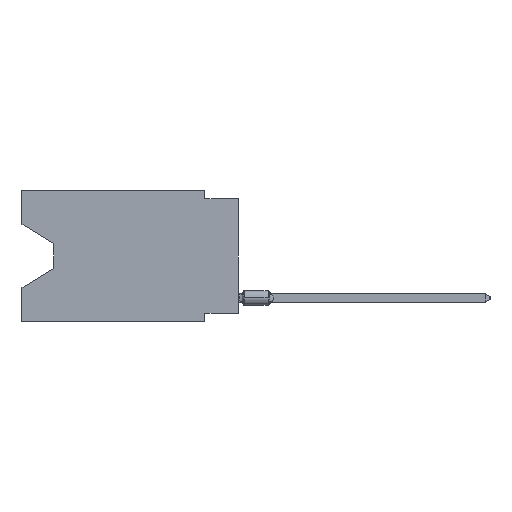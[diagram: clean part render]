
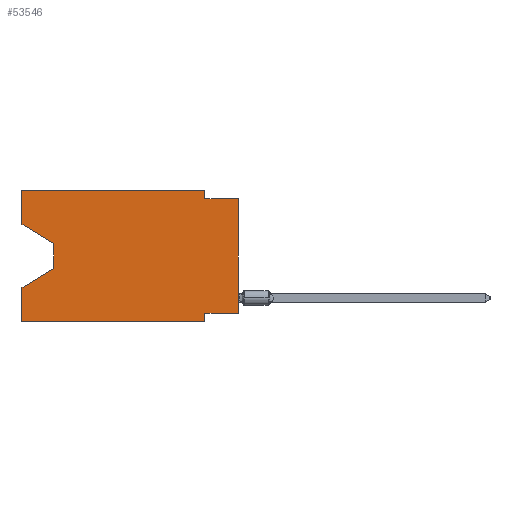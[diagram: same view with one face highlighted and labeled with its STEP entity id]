
A CAD part, left-side view. The second image highlights one B-rep face of the part: STEP entity #53546.
In plain terms, the highlighted planar face has unit normal (-1, 0, 0).
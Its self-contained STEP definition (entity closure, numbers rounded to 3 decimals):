
#423 = DIRECTION ( 'NONE',  ( 0., -1., 0. ) ) ;
#841 = ORIENTED_EDGE ( 'NONE', *, *, #26399, .T. ) ;
#1044 = CARTESIAN_POINT ( 'NONE',  ( 0., 16.383, 0. ) ) ;
#1350 = LINE ( 'NONE', #17742, #22564 ) ;
#1774 = DIRECTION ( 'NONE',  ( 0., 0., -1. ) ) ;
#2171 = VECTOR ( 'NONE', #1774, 1000. ) ;
#2993 = LINE ( 'NONE', #15288, #42739 ) ;
#4842 = CARTESIAN_POINT ( 'NONE',  ( 0., 16.383, 0. ) ) ;
#5201 = EDGE_CURVE ( 'NONE', #51063, #29394, #20993, .T. ) ;
#5454 = DIRECTION ( 'NONE',  ( 0., 0., 1. ) ) ;
#5623 = VERTEX_POINT ( 'NONE', #29862 ) ;
#5711 = CARTESIAN_POINT ( 'NONE',  ( 0., 2.54, 0. ) ) ;
#6202 = ORIENTED_EDGE ( 'NONE', *, *, #45270, .T. ) ;
#6523 = CARTESIAN_POINT ( 'NONE',  ( 0., 16.383, -7.36 ) ) ;
#6717 = EDGE_CURVE ( 'NONE', #31168, #6784, #40688, .T. ) ;
#6784 = VERTEX_POINT ( 'NONE', #37659 ) ;
#6823 = DIRECTION ( 'NONE',  ( 0., -0.855, -0.519 ) ) ;
#7343 = VECTOR ( 'NONE', #51184, 1000. ) ;
#7516 = LINE ( 'NONE', #15994, #32875 ) ;
#8274 = DIRECTION ( 'NONE',  ( 0., 0., -1. ) ) ;
#8316 = EDGE_CURVE ( 'NONE', #37069, #38059, #1350, .T. ) ;
#8361 = VECTOR ( 'NONE', #10678, 1000. ) ;
#8592 = VERTEX_POINT ( 'NONE', #14235 ) ;
#9373 = ORIENTED_EDGE ( 'NONE', *, *, #39799, .F. ) ;
#10678 = DIRECTION ( 'NONE',  ( 0., -1., 0. ) ) ;
#10828 = FACE_OUTER_BOUND ( 'NONE', #50442, .T. ) ;
#11593 = AXIS2_PLACEMENT_3D ( 'NONE', #39768, #43860, #23665 ) ;
#14235 = CARTESIAN_POINT ( 'NONE',  ( 0., 2.54, -9.271 ) ) ;
#15288 = CARTESIAN_POINT ( 'NONE',  ( 0., 2.54, 0. ) ) ;
#15776 = VECTOR ( 'NONE', #40937, 1000. ) ;
#15956 = LINE ( 'NONE', #16757, #31099 ) ;
#15994 = CARTESIAN_POINT ( 'NONE',  ( 0., 0., -9.271 ) ) ;
#16188 = CARTESIAN_POINT ( 'NONE',  ( 0., 16.383, 0. ) ) ;
#16381 = CARTESIAN_POINT ( 'NONE',  ( 0., 13.97, -5.893 ) ) ;
#16757 = CARTESIAN_POINT ( 'NONE',  ( 0., 13.97, -4.013 ) ) ;
#17003 = LINE ( 'NONE', #46170, #48349 ) ;
#17742 = CARTESIAN_POINT ( 'NONE',  ( 0., 16.383, 0. ) ) ;
#17753 = VERTEX_POINT ( 'NONE', #18349 ) ;
#18349 = CARTESIAN_POINT ( 'NONE',  ( 0., 13.97, -4.013 ) ) ;
#20993 = LINE ( 'NONE', #1044, #23973 ) ;
#21438 = CARTESIAN_POINT ( 'NONE',  ( 0., 16.383, -9.906 ) ) ;
#22564 = VECTOR ( 'NONE', #5454, 1000. ) ;
#23665 = DIRECTION ( 'NONE',  ( 0., 0., -1. ) ) ;
#23973 = VECTOR ( 'NONE', #37637, 1000. ) ;
#25239 = CARTESIAN_POINT ( 'NONE',  ( 0., 2.54, -9.906 ) ) ;
#25287 = ORIENTED_EDGE ( 'NONE', *, *, #6717, .F. ) ;
#26316 = EDGE_CURVE ( 'NONE', #51063, #17753, #51834, .T. ) ;
#26399 = EDGE_CURVE ( 'NONE', #5623, #38059, #28398, .T. ) ;
#27440 = ORIENTED_EDGE ( 'NONE', *, *, #5201, .F. ) ;
#28398 = LINE ( 'NONE', #16381, #15776 ) ;
#29394 = VERTEX_POINT ( 'NONE', #16188 ) ;
#29831 = ORIENTED_EDGE ( 'NONE', *, *, #8316, .F. ) ;
#29862 = CARTESIAN_POINT ( 'NONE',  ( 0., 13.97, -5.893 ) ) ;
#31099 = VECTOR ( 'NONE', #8274, 1000. ) ;
#31168 = VERTEX_POINT ( 'NONE', #50817 ) ;
#31726 = ORIENTED_EDGE ( 'NONE', *, *, #50036, .F. ) ;
#32007 = ORIENTED_EDGE ( 'NONE', *, *, #50470, .T. ) ;
#32875 = VECTOR ( 'NONE', #49506, 1000. ) ;
#32928 = ORIENTED_EDGE ( 'NONE', *, *, #46937, .T. ) ;
#33294 = VERTEX_POINT ( 'NONE', #45073 ) ;
#33722 = ORIENTED_EDGE ( 'NONE', *, *, #45146, .F. ) ;
#34260 = LINE ( 'NONE', #42992, #2171 ) ;
#37069 = VERTEX_POINT ( 'NONE', #39775 ) ;
#37253 = VERTEX_POINT ( 'NONE', #5711 ) ;
#37637 = DIRECTION ( 'NONE',  ( 0., 0., 1. ) ) ;
#37659 = CARTESIAN_POINT ( 'NONE',  ( 0., 0., -0.635 ) ) ;
#38059 = VERTEX_POINT ( 'NONE', #6523 ) ;
#39505 = PLANE ( 'NONE',  #11593 ) ;
#39629 = CARTESIAN_POINT ( 'NONE',  ( 0., 0., -0.635 ) ) ;
#39768 = CARTESIAN_POINT ( 'NONE',  ( 0., 16.383, 0. ) ) ;
#39775 = CARTESIAN_POINT ( 'NONE',  ( 0., 16.383, -9.906 ) ) ;
#39799 = EDGE_CURVE ( 'NONE', #33294, #8592, #7516, .T. ) ;
#39873 = CARTESIAN_POINT ( 'NONE',  ( 0., 16.383, -2.546 ) ) ;
#40040 = VERTEX_POINT ( 'NONE', #25239 ) ;
#40342 = ORIENTED_EDGE ( 'NONE', *, *, #26316, .T. ) ;
#40688 = LINE ( 'NONE', #39629, #8361 ) ;
#40937 = DIRECTION ( 'NONE',  ( 0., 0.855, -0.519 ) ) ;
#42355 = ORIENTED_EDGE ( 'NONE', *, *, #52744, .F. ) ;
#42651 = CARTESIAN_POINT ( 'NONE',  ( 0., 16.383, -2.546 ) ) ;
#42739 = VECTOR ( 'NONE', #45001, 1000. ) ;
#42992 = CARTESIAN_POINT ( 'NONE',  ( 0., 2.54, -9.906 ) ) ;
#43860 = DIRECTION ( 'NONE',  ( 1., 0., 0. ) ) ;
#45001 = DIRECTION ( 'NONE',  ( 0., 0., -1. ) ) ;
#45073 = CARTESIAN_POINT ( 'NONE',  ( 0., 0., -9.271 ) ) ;
#45146 = EDGE_CURVE ( 'NONE', #8592, #40040, #34260, .T. ) ;
#45270 = EDGE_CURVE ( 'NONE', #33294, #6784, #17003, .T. ) ;
#45838 = VECTOR ( 'NONE', #423, 1000. ) ;
#45990 = LINE ( 'NONE', #21438, #45838 ) ;
#46170 = CARTESIAN_POINT ( 'NONE',  ( 0., 0., 0. ) ) ;
#46937 = EDGE_CURVE ( 'NONE', #17753, #5623, #15956, .T. ) ;
#47128 = LINE ( 'NONE', #4842, #7343 ) ;
#48349 = VECTOR ( 'NONE', #49980, 1000. ) ;
#49506 = DIRECTION ( 'NONE',  ( 0., 1., 0. ) ) ;
#49980 = DIRECTION ( 'NONE',  ( 0., 0., 1. ) ) ;
#50036 = EDGE_CURVE ( 'NONE', #29394, #37253, #47128, .T. ) ;
#50442 = EDGE_LOOP ( 'NONE', ( #40342, #32928, #841, #29831, #32007, #33722, #9373, #6202, #25287, #42355, #31726, #27440 ) ) ;
#50470 = EDGE_CURVE ( 'NONE', #37069, #40040, #45990, .T. ) ;
#50817 = CARTESIAN_POINT ( 'NONE',  ( 0., 2.54, -0.635 ) ) ;
#51063 = VERTEX_POINT ( 'NONE', #42651 ) ;
#51184 = DIRECTION ( 'NONE',  ( 0., -1., 0. ) ) ;
#51834 = LINE ( 'NONE', #39873, #53015 ) ;
#52744 = EDGE_CURVE ( 'NONE', #37253, #31168, #2993, .T. ) ;
#53015 = VECTOR ( 'NONE', #6823, 1000. ) ;
#53546 = ADVANCED_FACE ( 'NONE', ( #10828 ), #39505, .F. ) ;
